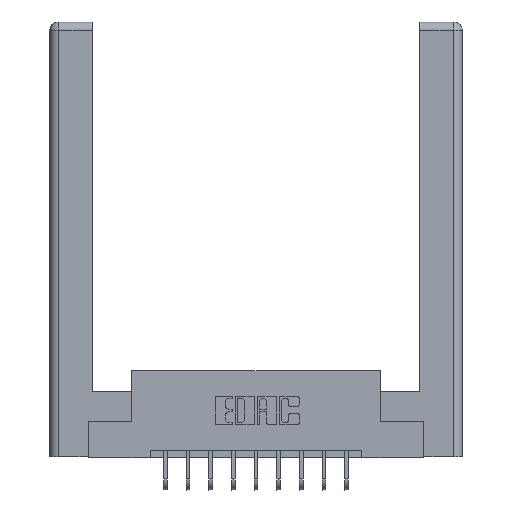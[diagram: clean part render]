
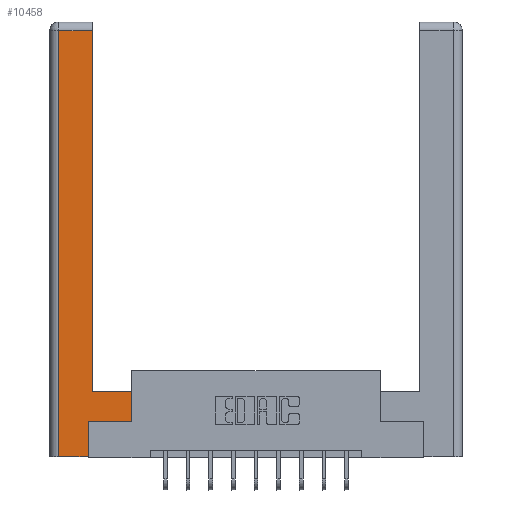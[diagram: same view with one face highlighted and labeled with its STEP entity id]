
A CAD part, top view. The second image highlights one B-rep face of the part: STEP entity #10458.
In plain terms, the highlighted planar face has unit normal (0, 0, 1).
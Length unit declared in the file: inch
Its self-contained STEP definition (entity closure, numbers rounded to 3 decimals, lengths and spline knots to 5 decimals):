
#97 = AXIS2_PLACEMENT_3D ( 'NONE', #907, #7075, #11870 ) ;
#431 = ORIENTED_EDGE ( 'NONE', *, *, #1996, .T. ) ;
#474 = VERTEX_POINT ( 'NONE', #15255 ) ;
#590 = VERTEX_POINT ( 'NONE', #12048 ) ;
#907 = CARTESIAN_POINT ( 'NONE',  ( 0., 0., 0. ) ) ;
#1016 = PLANE ( 'NONE',  #97 ) ;
#1661 = VECTOR ( 'NONE', #5468, 39.37008 ) ;
#1996 = EDGE_CURVE ( 'NONE', #6886, #5013, #7647, .T. ) ;
#2224 = VERTEX_POINT ( 'NONE', #4954 ) ;
#2307 = LINE ( 'NONE', #8684, #11970 ) ;
#2567 = VERTEX_POINT ( 'NONE', #7030 ) ;
#3025 = DIRECTION ( 'NONE',  ( 0., 1., 0. ) ) ;
#3084 = DIRECTION ( 'NONE',  ( -1., 0., 0. ) ) ;
#3334 = LINE ( 'NONE', #4837, #14135 ) ;
#3510 = EDGE_CURVE ( 'NONE', #2567, #6886, #2307, .T. ) ;
#3729 = VECTOR ( 'NONE', #7337, 39.37008 ) ;
#3783 = LINE ( 'NONE', #9294, #5117 ) ;
#3927 = LINE ( 'NONE', #15299, #3729 ) ;
#4301 = ORIENTED_EDGE ( 'NONE', *, *, #14969, .T. ) ;
#4756 = ORIENTED_EDGE ( 'NONE', *, *, #3510, .T. ) ;
#4837 = CARTESIAN_POINT ( 'NONE',  ( 0.265, 0.245, 0. ) ) ;
#4954 = CARTESIAN_POINT ( 'NONE',  ( 0.0615, 0., 0. ) ) ;
#5013 = VERTEX_POINT ( 'NONE', #11166 ) ;
#5117 = VECTOR ( 'NONE', #15394, 39.37008 ) ;
#5430 = ORIENTED_EDGE ( 'NONE', *, *, #7490, .T. ) ;
#5468 = DIRECTION ( 'NONE',  ( 1., 0., 0. ) ) ;
#5550 = DIRECTION ( 'NONE',  ( 0., 1., 0. ) ) ;
#5916 = EDGE_CURVE ( 'NONE', #10879, #2567, #3334, .T. ) ;
#6348 = CARTESIAN_POINT ( 'NONE',  ( 0.0615, 2.94, 0. ) ) ;
#6442 = CARTESIAN_POINT ( 'NONE',  ( 0.265, 0., 0. ) ) ;
#6886 = VERTEX_POINT ( 'NONE', #12267 ) ;
#7030 = CARTESIAN_POINT ( 'NONE',  ( 0.265, 0.245, 0. ) ) ;
#7075 = DIRECTION ( 'NONE',  ( 0., 0., -1. ) ) ;
#7337 = DIRECTION ( 'NONE',  ( 0., -1., 0. ) ) ;
#7490 = EDGE_CURVE ( 'NONE', #2224, #10879, #11521, .T. ) ;
#7647 = LINE ( 'NONE', #11549, #14831 ) ;
#7842 = EDGE_LOOP ( 'NONE', ( #9721, #4301, #7951, #5430, #13484, #4756, #431, #15155 ) ) ;
#7918 = VECTOR ( 'NONE', #12649, 39.37008 ) ;
#7951 = ORIENTED_EDGE ( 'NONE', *, *, #8316, .T. ) ;
#8316 = EDGE_CURVE ( 'NONE', #15460, #2224, #3927, .T. ) ;
#8684 = CARTESIAN_POINT ( 'NONE',  ( 0.565, 0.245, 0. ) ) ;
#9294 = CARTESIAN_POINT ( 'NONE',  ( 0.0615, 2.94, 0. ) ) ;
#9721 = ORIENTED_EDGE ( 'NONE', *, *, #14838, .T. ) ;
#10198 = CARTESIAN_POINT ( 'NONE',  ( 0.295, 3., 0. ) ) ;
#10458 = ADVANCED_FACE ( 'NONE', ( #15413 ), #1016, .F. ) ;
#10879 = VERTEX_POINT ( 'NONE', #6442 ) ;
#10975 = LINE ( 'NONE', #15184, #14763 ) ;
#11166 = CARTESIAN_POINT ( 'NONE',  ( 0.565, 0.45, 0. ) ) ;
#11521 = LINE ( 'NONE', #15058, #1661 ) ;
#11549 = CARTESIAN_POINT ( 'NONE',  ( 0.565, 0.45, 0. ) ) ;
#11870 = DIRECTION ( 'NONE',  ( -1., 0., 0. ) ) ;
#11970 = VECTOR ( 'NONE', #12196, 39.37008 ) ;
#12048 = CARTESIAN_POINT ( 'NONE',  ( 0.295, 2.94, 0. ) ) ;
#12196 = DIRECTION ( 'NONE',  ( 1., 0., 0. ) ) ;
#12267 = CARTESIAN_POINT ( 'NONE',  ( 0.565, 0.245, 0. ) ) ;
#12649 = DIRECTION ( 'NONE',  ( 0., 1., 0. ) ) ;
#13484 = ORIENTED_EDGE ( 'NONE', *, *, #5916, .T. ) ;
#14135 = VECTOR ( 'NONE', #5550, 39.37008 ) ;
#14581 = EDGE_CURVE ( 'NONE', #5013, #474, #10975, .T. ) ;
#14763 = VECTOR ( 'NONE', #3084, 39.37008 ) ;
#14831 = VECTOR ( 'NONE', #3025, 39.37008 ) ;
#14838 = EDGE_CURVE ( 'NONE', #474, #590, #15490, .T. ) ;
#14969 = EDGE_CURVE ( 'NONE', #590, #15460, #3783, .T. ) ;
#15058 = CARTESIAN_POINT ( 'NONE',  ( 0.265, 0., 0. ) ) ;
#15155 = ORIENTED_EDGE ( 'NONE', *, *, #14581, .T. ) ;
#15184 = CARTESIAN_POINT ( 'NONE',  ( 0.295, 0.45, 0. ) ) ;
#15255 = CARTESIAN_POINT ( 'NONE',  ( 0.295, 0.45, 0. ) ) ;
#15299 = CARTESIAN_POINT ( 'NONE',  ( 0.0615, 0., 0. ) ) ;
#15394 = DIRECTION ( 'NONE',  ( -1., 0., 0. ) ) ;
#15413 = FACE_OUTER_BOUND ( 'NONE', #7842, .T. ) ;
#15460 = VERTEX_POINT ( 'NONE', #6348 ) ;
#15490 = LINE ( 'NONE', #10198, #7918 ) ;
